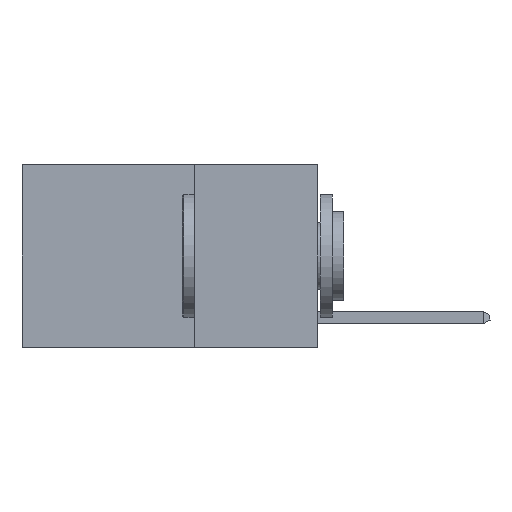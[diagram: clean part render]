
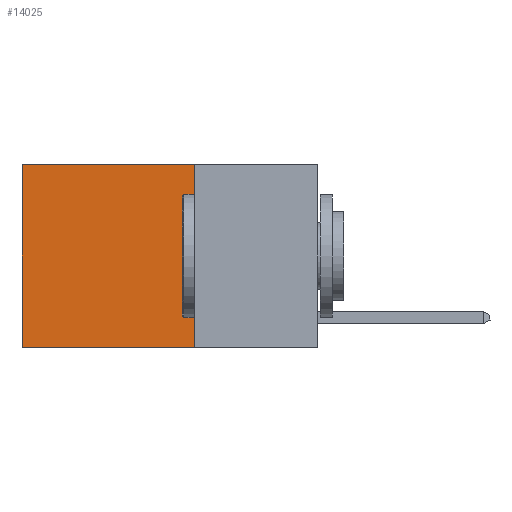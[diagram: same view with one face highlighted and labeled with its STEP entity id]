
A CAD part, left-side view. The second image highlights one B-rep face of the part: STEP entity #14025.
In plain terms, the highlighted planar face has unit normal (-1, 0, 0).
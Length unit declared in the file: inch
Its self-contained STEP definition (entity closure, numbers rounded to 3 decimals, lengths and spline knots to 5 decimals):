
#1243 = EDGE_CURVE ( 'NONE', #8831, #9865, #15697, .T. ) ;
#1653 = DIRECTION ( 'NONE',  ( 1., 0., 0. ) ) ;
#2297 = LINE ( 'NONE', #5209, #23396 ) ;
#3381 = VECTOR ( 'NONE', #16706, 39.37008 ) ;
#5209 = CARTESIAN_POINT ( 'NONE',  ( 0.2625, 0.25, -0.37 ) ) ;
#5794 = CARTESIAN_POINT ( 'NONE',  ( 0.2625, 0.6, -0.37 ) ) ;
#6364 = VECTOR ( 'NONE', #7219, 39.37008 ) ;
#7219 = DIRECTION ( 'NONE',  ( 0., 0., -1. ) ) ;
#7528 = AXIS2_PLACEMENT_3D ( 'NONE', #10114, #1653, #16515 ) ;
#8022 = PLANE ( 'NONE',  #7528 ) ;
#8684 = CARTESIAN_POINT ( 'NONE',  ( 0.2625, 0.6, 0. ) ) ;
#8831 = VERTEX_POINT ( 'NONE', #8684 ) ;
#9181 = FACE_OUTER_BOUND ( 'NONE', #21959, .T. ) ;
#9865 = VERTEX_POINT ( 'NONE', #5794 ) ;
#10062 = VECTOR ( 'NONE', #19657, 39.37008 ) ;
#10114 = CARTESIAN_POINT ( 'NONE',  ( 0.2625, 0.25, 0. ) ) ;
#10570 = ORIENTED_EDGE ( 'NONE', *, *, #23784, .F. ) ;
#11336 = LINE ( 'NONE', #19832, #6364 ) ;
#11758 = CARTESIAN_POINT ( 'NONE',  ( 0.2625, 0.25, -0.37 ) ) ;
#11909 = ORIENTED_EDGE ( 'NONE', *, *, #15969, .T. ) ;
#12209 = VERTEX_POINT ( 'NONE', #23189 ) ;
#14025 = ADVANCED_FACE ( 'NONE', ( #9181 ), #8022, .F. ) ;
#15697 = LINE ( 'NONE', #17556, #10062 ) ;
#15969 = EDGE_CURVE ( 'NONE', #12209, #8831, #25753, .T. ) ;
#16515 = DIRECTION ( 'NONE',  ( 0., 0., -1. ) ) ;
#16706 = DIRECTION ( 'NONE',  ( 0., 1., 0. ) ) ;
#17556 = CARTESIAN_POINT ( 'NONE',  ( 0.2625, 0.6, 0. ) ) ;
#17893 = DIRECTION ( 'NONE',  ( 0., 1., 0. ) ) ;
#18351 = ORIENTED_EDGE ( 'NONE', *, *, #1243, .T. ) ;
#19657 = DIRECTION ( 'NONE',  ( 0., 0., -1. ) ) ;
#19796 = VERTEX_POINT ( 'NONE', #11758 ) ;
#19832 = CARTESIAN_POINT ( 'NONE',  ( 0.2625, 0.25, 0. ) ) ;
#21959 = EDGE_LOOP ( 'NONE', ( #18351, #10570, #24136, #11909 ) ) ;
#23176 = EDGE_CURVE ( 'NONE', #12209, #19796, #11336, .T. ) ;
#23189 = CARTESIAN_POINT ( 'NONE',  ( 0.2625, 0.25, 0. ) ) ;
#23396 = VECTOR ( 'NONE', #17893, 39.37008 ) ;
#23784 = EDGE_CURVE ( 'NONE', #19796, #9865, #2297, .T. ) ;
#24136 = ORIENTED_EDGE ( 'NONE', *, *, #23176, .F. ) ;
#25753 = LINE ( 'NONE', #27084, #3381 ) ;
#27084 = CARTESIAN_POINT ( 'NONE',  ( 0.2625, 0.25, 0. ) ) ;
